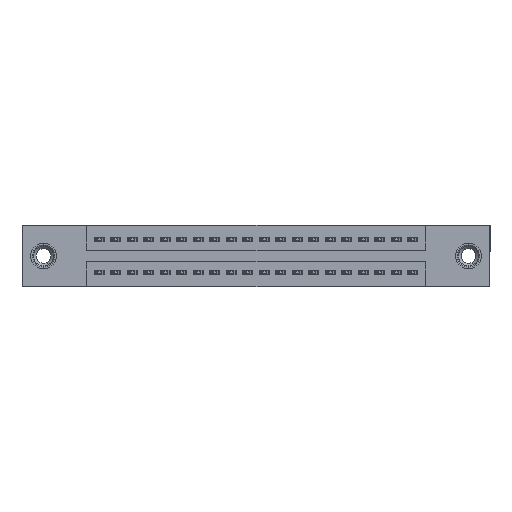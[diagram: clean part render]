
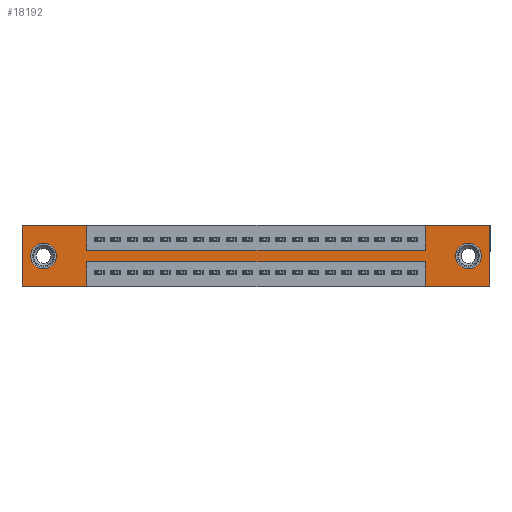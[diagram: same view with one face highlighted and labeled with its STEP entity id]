
A CAD part, front view. The second image highlights one B-rep face of the part: STEP entity #18192.
In plain terms, the highlighted planar face has unit normal (0, -1, 0).
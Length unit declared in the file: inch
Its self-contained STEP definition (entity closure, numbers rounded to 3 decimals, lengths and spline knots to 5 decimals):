
#271 = CARTESIAN_POINT ( 'NONE',  ( 2.4425, 0., -0.37 ) ) ;
#1070 = DIRECTION ( 'NONE',  ( 0., 0., 1. ) ) ;
#1189 = CARTESIAN_POINT ( 'NONE',  ( 0.3925, 0., 0. ) ) ;
#1387 = VECTOR ( 'NONE', #16857, 39.37008 ) ;
#1512 = VECTOR ( 'NONE', #8653, 39.37008 ) ;
#1577 = CIRCLE ( 'NONE', #11760, 0.078 ) ;
#1956 = LINE ( 'NONE', #10711, #6004 ) ;
#1962 = EDGE_CURVE ( 'NONE', #17293, #8360, #19675, .T. ) ;
#2078 = DIRECTION ( 'NONE',  ( 0., 0., 1. ) ) ;
#2108 = CARTESIAN_POINT ( 'NONE',  ( 0.13, 0., -0.263 ) ) ;
#2385 = ORIENTED_EDGE ( 'NONE', *, *, #11731, .F. ) ;
#2611 = EDGE_CURVE ( 'NONE', #12689, #16087, #15820, .T. ) ;
#2730 = DIRECTION ( 'NONE',  ( -1., 0., 0. ) ) ;
#2894 = EDGE_CURVE ( 'NONE', #7103, #7840, #13775, .T. ) ;
#2904 = VECTOR ( 'NONE', #1070, 39.37008 ) ;
#3065 = EDGE_LOOP ( 'NONE', ( #14916, #11078 ) ) ;
#3078 = CARTESIAN_POINT ( 'NONE',  ( 2.835, 0., -0.37 ) ) ;
#3186 = ORIENTED_EDGE ( 'NONE', *, *, #10038, .F. ) ;
#3303 = VECTOR ( 'NONE', #10809, 39.37008 ) ;
#3681 = DIRECTION ( 'NONE',  ( 0., 0., 1. ) ) ;
#3791 = EDGE_CURVE ( 'NONE', #8637, #10365, #5989, .T. ) ;
#4004 = DIRECTION ( 'NONE',  ( 0., 1., 0. ) ) ;
#4181 = EDGE_LOOP ( 'NONE', ( #14765, #20080 ) ) ;
#4456 = CARTESIAN_POINT ( 'NONE',  ( 0., 0., 0. ) ) ;
#4534 = CARTESIAN_POINT ( 'NONE',  ( 0.13, 0., -0.107 ) ) ;
#4536 = CARTESIAN_POINT ( 'NONE',  ( 2.835, 0., 0. ) ) ;
#4812 = VERTEX_POINT ( 'NONE', #5377 ) ;
#5211 = CARTESIAN_POINT ( 'NONE',  ( 0., 0., -0.37 ) ) ;
#5323 = DIRECTION ( 'NONE',  ( 1., 0., 0. ) ) ;
#5377 = CARTESIAN_POINT ( 'NONE',  ( 2.4425, 0., 0. ) ) ;
#5418 = DIRECTION ( 'NONE',  ( 0., 0., -1. ) ) ;
#5447 = ORIENTED_EDGE ( 'NONE', *, *, #8347, .F. ) ;
#5518 = CARTESIAN_POINT ( 'NONE',  ( 0.3925, 0., -0.15 ) ) ;
#5536 = VECTOR ( 'NONE', #16457, 39.37008 ) ;
#5538 = CARTESIAN_POINT ( 'NONE',  ( 0., 0., -0.37 ) ) ;
#5652 = LINE ( 'NONE', #18425, #1387 ) ;
#5989 = CIRCLE ( 'NONE', #18691, 0.078 ) ;
#6004 = VECTOR ( 'NONE', #9043, 39.37008 ) ;
#6519 = FACE_OUTER_BOUND ( 'NONE', #18972, .T. ) ;
#6852 = CARTESIAN_POINT ( 'NONE',  ( 0.3925, 0., -0.15 ) ) ;
#6997 = CARTESIAN_POINT ( 'NONE',  ( 2.4425, 0., -0.37 ) ) ;
#7103 = VERTEX_POINT ( 'NONE', #16591 ) ;
#7149 = VERTEX_POINT ( 'NONE', #18579 ) ;
#7210 = CARTESIAN_POINT ( 'NONE',  ( 0.3925, 0., -0.37 ) ) ;
#7281 = CARTESIAN_POINT ( 'NONE',  ( 2.705, 0., -0.185 ) ) ;
#7540 = VECTOR ( 'NONE', #12833, 39.37008 ) ;
#7723 = VERTEX_POINT ( 'NONE', #9153 ) ;
#7840 = VERTEX_POINT ( 'NONE', #7210 ) ;
#7986 = AXIS2_PLACEMENT_3D ( 'NONE', #7281, #16690, #5418 ) ;
#8117 = EDGE_CURVE ( 'NONE', #7840, #7723, #14174, .T. ) ;
#8201 = ORIENTED_EDGE ( 'NONE', *, *, #2894, .F. ) ;
#8304 = CARTESIAN_POINT ( 'NONE',  ( 0.3925, 0., -0.37 ) ) ;
#8347 = EDGE_CURVE ( 'NONE', #7149, #7103, #13117, .T. ) ;
#8360 = VERTEX_POINT ( 'NONE', #16898 ) ;
#8515 = LINE ( 'NONE', #18267, #1512 ) ;
#8637 = VERTEX_POINT ( 'NONE', #2108 ) ;
#8653 = DIRECTION ( 'NONE',  ( 0., 0., 1. ) ) ;
#8695 = DIRECTION ( 'NONE',  ( 0., 0., 1. ) ) ;
#8956 = ORIENTED_EDGE ( 'NONE', *, *, #18754, .F. ) ;
#9043 = DIRECTION ( 'NONE',  ( 1., 0., 0. ) ) ;
#9153 = CARTESIAN_POINT ( 'NONE',  ( 0., 0., -0.37 ) ) ;
#9290 = LINE ( 'NONE', #20804, #7540 ) ;
#9865 = ORIENTED_EDGE ( 'NONE', *, *, #8117, .F. ) ;
#9877 = ORIENTED_EDGE ( 'NONE', *, *, #20575, .F. ) ;
#10038 = EDGE_CURVE ( 'NONE', #18651, #13749, #17850, .T. ) ;
#10087 = CARTESIAN_POINT ( 'NONE',  ( 2.835, 0., 0. ) ) ;
#10365 = VERTEX_POINT ( 'NONE', #4534 ) ;
#10416 = LINE ( 'NONE', #14007, #2904 ) ;
#10417 = EDGE_CURVE ( 'NONE', #16087, #12689, #11293, .T. ) ;
#10551 = ORIENTED_EDGE ( 'NONE', *, *, #11412, .F. ) ;
#10711 = CARTESIAN_POINT ( 'NONE',  ( 0., 0., 0. ) ) ;
#10809 = DIRECTION ( 'NONE',  ( 0., 0., -1. ) ) ;
#10860 = EDGE_CURVE ( 'NONE', #11974, #17293, #9290, .T. ) ;
#11067 = VECTOR ( 'NONE', #5323, 39.37008 ) ;
#11078 = ORIENTED_EDGE ( 'NONE', *, *, #3791, .T. ) ;
#11235 = DIRECTION ( 'NONE',  ( 0., 1., 0. ) ) ;
#11293 = CIRCLE ( 'NONE', #7986, 0.078 ) ;
#11366 = CARTESIAN_POINT ( 'NONE',  ( 2.705, 0., -0.185 ) ) ;
#11412 = EDGE_CURVE ( 'NONE', #8360, #4812, #8515, .T. ) ;
#11625 = VECTOR ( 'NONE', #2730, 39.37008 ) ;
#11731 = EDGE_CURVE ( 'NONE', #13592, #7149, #18095, .T. ) ;
#11760 = AXIS2_PLACEMENT_3D ( 'NONE', #18049, #19736, #3681 ) ;
#11772 = CARTESIAN_POINT ( 'NONE',  ( 2.705, 0., -0.263 ) ) ;
#11918 = VECTOR ( 'NONE', #16420, 39.37008 ) ;
#11974 = VERTEX_POINT ( 'NONE', #1189 ) ;
#12447 = CARTESIAN_POINT ( 'NONE',  ( 2.705, 0., -0.107 ) ) ;
#12689 = VERTEX_POINT ( 'NONE', #12447 ) ;
#12833 = DIRECTION ( 'NONE',  ( 0., 0., -1. ) ) ;
#12839 = DIRECTION ( 'NONE',  ( 0., 0., -1. ) ) ;
#13117 = LINE ( 'NONE', #15482, #11625 ) ;
#13535 = DIRECTION ( 'NONE',  ( -1., 0., 0. ) ) ;
#13592 = VERTEX_POINT ( 'NONE', #271 ) ;
#13749 = VERTEX_POINT ( 'NONE', #3078 ) ;
#13775 = LINE ( 'NONE', #8304, #5536 ) ;
#13811 = VECTOR ( 'NONE', #2078, 39.37008 ) ;
#14007 = CARTESIAN_POINT ( 'NONE',  ( 0., 0., 0. ) ) ;
#14029 = PLANE ( 'NONE',  #19098 ) ;
#14174 = LINE ( 'NONE', #5538, #17195 ) ;
#14765 = ORIENTED_EDGE ( 'NONE', *, *, #2611, .T. ) ;
#14916 = ORIENTED_EDGE ( 'NONE', *, *, #17645, .T. ) ;
#15097 = EDGE_CURVE ( 'NONE', #15952, #11974, #5652, .T. ) ;
#15447 = ORIENTED_EDGE ( 'NONE', *, *, #10860, .F. ) ;
#15482 = CARTESIAN_POINT ( 'NONE',  ( 0.3925, 0., -0.22 ) ) ;
#15799 = FACE_BOUND ( 'NONE', #3065, .T. ) ;
#15820 = CIRCLE ( 'NONE', #17305, 0.078 ) ;
#15952 = VERTEX_POINT ( 'NONE', #4456 ) ;
#16072 = ORIENTED_EDGE ( 'NONE', *, *, #1962, .F. ) ;
#16087 = VERTEX_POINT ( 'NONE', #11772 ) ;
#16420 = DIRECTION ( 'NONE',  ( -1., 0., 0. ) ) ;
#16457 = DIRECTION ( 'NONE',  ( 0., 0., -1. ) ) ;
#16591 = CARTESIAN_POINT ( 'NONE',  ( 0.3925, 0., -0.22 ) ) ;
#16690 = DIRECTION ( 'NONE',  ( 0., 1., 0. ) ) ;
#16709 = LINE ( 'NONE', #5211, #11918 ) ;
#16857 = DIRECTION ( 'NONE',  ( 1., 0., 0. ) ) ;
#16898 = CARTESIAN_POINT ( 'NONE',  ( 2.4425, 0., -0.15 ) ) ;
#17195 = VECTOR ( 'NONE', #13535, 39.37008 ) ;
#17293 = VERTEX_POINT ( 'NONE', #5518 ) ;
#17305 = AXIS2_PLACEMENT_3D ( 'NONE', #11366, #11235, #12839 ) ;
#17345 = CARTESIAN_POINT ( 'NONE',  ( 0., 0., -0.37 ) ) ;
#17451 = ORIENTED_EDGE ( 'NONE', *, *, #15097, .F. ) ;
#17645 = EDGE_CURVE ( 'NONE', #10365, #8637, #1577, .T. ) ;
#17850 = LINE ( 'NONE', #4536, #3303 ) ;
#18049 = CARTESIAN_POINT ( 'NONE',  ( 0.13, 0., -0.185 ) ) ;
#18095 = LINE ( 'NONE', #6997, #13811 ) ;
#18192 = ADVANCED_FACE ( 'NONE', ( #20151, #15799, #6519 ), #14029, .T. ) ;
#18267 = CARTESIAN_POINT ( 'NONE',  ( 2.4425, 0., 0. ) ) ;
#18425 = CARTESIAN_POINT ( 'NONE',  ( 0., 0., 0. ) ) ;
#18452 = ORIENTED_EDGE ( 'NONE', *, *, #20809, .F. ) ;
#18579 = CARTESIAN_POINT ( 'NONE',  ( 2.4425, 0., -0.22 ) ) ;
#18604 = CARTESIAN_POINT ( 'NONE',  ( 0.13, 0., -0.185 ) ) ;
#18651 = VERTEX_POINT ( 'NONE', #10087 ) ;
#18691 = AXIS2_PLACEMENT_3D ( 'NONE', #18604, #4004, #8695 ) ;
#18754 = EDGE_CURVE ( 'NONE', #4812, #18651, #1956, .T. ) ;
#18796 = DIRECTION ( 'NONE',  ( 0., 0., -1. ) ) ;
#18972 = EDGE_LOOP ( 'NONE', ( #8201, #5447, #2385, #9877, #3186, #8956, #10551, #16072, #15447, #17451, #18452, #9865 ) ) ;
#19008 = DIRECTION ( 'NONE',  ( 0., -1., 0. ) ) ;
#19098 = AXIS2_PLACEMENT_3D ( 'NONE', #17345, #19008, #18796 ) ;
#19675 = LINE ( 'NONE', #6852, #11067 ) ;
#19736 = DIRECTION ( 'NONE',  ( 0., 1., 0. ) ) ;
#20080 = ORIENTED_EDGE ( 'NONE', *, *, #10417, .T. ) ;
#20151 = FACE_BOUND ( 'NONE', #4181, .T. ) ;
#20575 = EDGE_CURVE ( 'NONE', #13749, #13592, #16709, .T. ) ;
#20804 = CARTESIAN_POINT ( 'NONE',  ( 0.3925, 0., 0. ) ) ;
#20809 = EDGE_CURVE ( 'NONE', #7723, #15952, #10416, .T. ) ;
